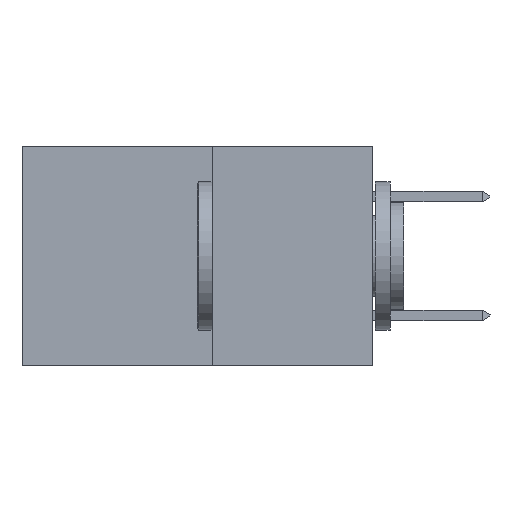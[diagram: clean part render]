
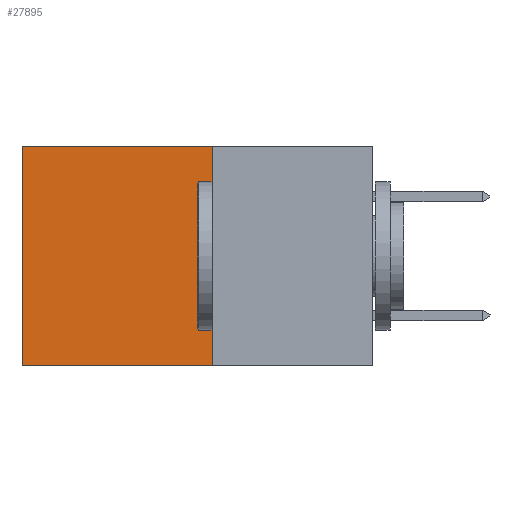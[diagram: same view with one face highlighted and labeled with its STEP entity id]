
A CAD part, left-side view. The second image highlights one B-rep face of the part: STEP entity #27895.
In plain terms, the highlighted planar face has unit normal (-1, 0, 0).
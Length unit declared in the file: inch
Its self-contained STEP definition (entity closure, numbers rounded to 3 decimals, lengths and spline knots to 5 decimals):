
#795 = CARTESIAN_POINT ( 'NONE',  ( 0.277, 0.27, 0. ) ) ;
#857 = DIRECTION ( 'NONE',  ( 0., 0., -1. ) ) ;
#1181 = VERTEX_POINT ( 'NONE', #18817 ) ;
#1392 = DIRECTION ( 'NONE',  ( 1., 0., 0. ) ) ;
#1441 = EDGE_CURVE ( 'NONE', #1181, #20555, #14469, .T. ) ;
#1870 = CARTESIAN_POINT ( 'NONE',  ( 0.277, 0.59, -0.37 ) ) ;
#2627 = CARTESIAN_POINT ( 'NONE',  ( 0.277, 0.59, -0.37 ) ) ;
#4398 = DIRECTION ( 'NONE',  ( 0., 0., -1. ) ) ;
#4839 = FACE_OUTER_BOUND ( 'NONE', #30980, .T. ) ;
#4875 = VECTOR ( 'NONE', #4398, 39.37008 ) ;
#5664 = LINE ( 'NONE', #1870, #4875 ) ;
#8203 = VECTOR ( 'NONE', #15928, 39.37008 ) ;
#8480 = CARTESIAN_POINT ( 'NONE',  ( 0.277, 0.27, -0.37 ) ) ;
#8567 = VECTOR ( 'NONE', #28781, 39.37008 ) ;
#8819 = LINE ( 'NONE', #8480, #22308 ) ;
#10773 = CARTESIAN_POINT ( 'NONE',  ( 0.277, 0.27, -0.37 ) ) ;
#11420 = ORIENTED_EDGE ( 'NONE', *, *, #27768, .F. ) ;
#11427 = CARTESIAN_POINT ( 'NONE',  ( 0.277, 0.27, -0.37 ) ) ;
#13832 = CARTESIAN_POINT ( 'NONE',  ( 0.277, 0.27, 0. ) ) ;
#13995 = EDGE_CURVE ( 'NONE', #32069, #14101, #27656, .T. ) ;
#14101 = VERTEX_POINT ( 'NONE', #23935 ) ;
#14469 = LINE ( 'NONE', #10773, #8567 ) ;
#15541 = ORIENTED_EDGE ( 'NONE', *, *, #13995, .T. ) ;
#15928 = DIRECTION ( 'NONE',  ( 0., 1., 0. ) ) ;
#18817 = CARTESIAN_POINT ( 'NONE',  ( 0.277, 0.27, -0.37 ) ) ;
#19074 = DIRECTION ( 'NONE',  ( 0., 0., -1. ) ) ;
#20555 = VERTEX_POINT ( 'NONE', #2627 ) ;
#21543 = PLANE ( 'NONE',  #29043 ) ;
#22308 = VECTOR ( 'NONE', #857, 39.37008 ) ;
#23520 = ORIENTED_EDGE ( 'NONE', *, *, #1441, .F. ) ;
#23935 = CARTESIAN_POINT ( 'NONE',  ( 0.277, 0.59, 0. ) ) ;
#26853 = ORIENTED_EDGE ( 'NONE', *, *, #27425, .T. ) ;
#27425 = EDGE_CURVE ( 'NONE', #14101, #20555, #5664, .T. ) ;
#27656 = LINE ( 'NONE', #795, #8203 ) ;
#27768 = EDGE_CURVE ( 'NONE', #32069, #1181, #8819, .T. ) ;
#27895 = ADVANCED_FACE ( 'NONE', ( #4839 ), #21543, .F. ) ;
#28781 = DIRECTION ( 'NONE',  ( 0., 1., 0. ) ) ;
#29043 = AXIS2_PLACEMENT_3D ( 'NONE', #11427, #1392, #19074 ) ;
#30980 = EDGE_LOOP ( 'NONE', ( #26853, #23520, #11420, #15541 ) ) ;
#32069 = VERTEX_POINT ( 'NONE', #13832 ) ;
